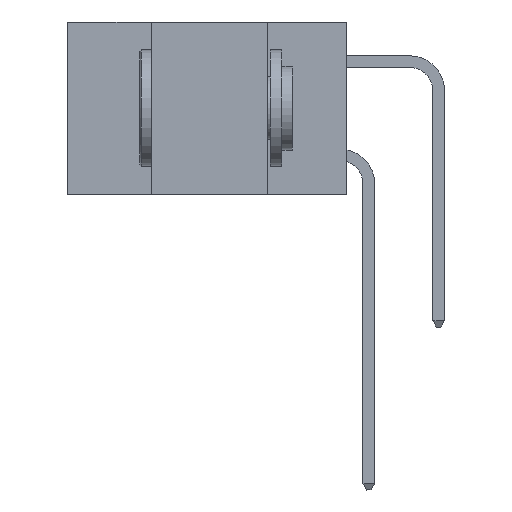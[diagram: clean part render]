
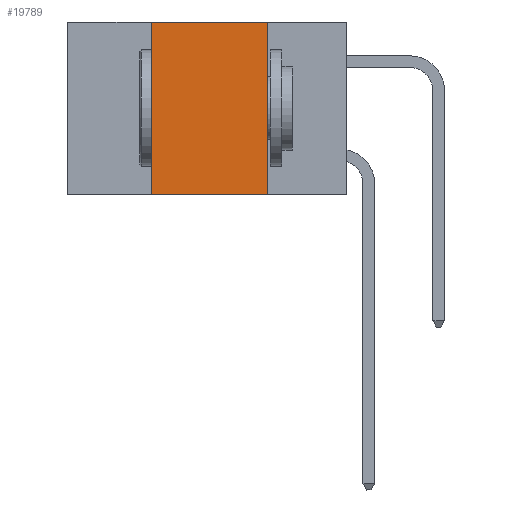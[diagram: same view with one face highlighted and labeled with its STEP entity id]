
A CAD part, left-side view. The second image highlights one B-rep face of the part: STEP entity #19789.
In plain terms, the highlighted planar face has unit normal (-1, 0, 0).
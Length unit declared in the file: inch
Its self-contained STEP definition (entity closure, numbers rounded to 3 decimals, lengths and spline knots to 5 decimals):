
#940 = VERTEX_POINT ( 'NONE', #16587 ) ;
#1524 = EDGE_LOOP ( 'NONE', ( #10080, #21370, #4394, #13162 ) ) ;
#1632 = VERTEX_POINT ( 'NONE', #16380 ) ;
#4146 = LINE ( 'NONE', #13945, #11488 ) ;
#4394 = ORIENTED_EDGE ( 'NONE', *, *, #10750, .F. ) ;
#5174 = DIRECTION ( 'NONE',  ( 0., 0., 1. ) ) ;
#5801 = DIRECTION ( 'NONE',  ( 0., 0., -1. ) ) ;
#6802 = LINE ( 'NONE', #19123, #24147 ) ;
#8670 = CARTESIAN_POINT ( 'NONE',  ( 0., 0.6, -0.37 ) ) ;
#10080 = ORIENTED_EDGE ( 'NONE', *, *, #20058, .F. ) ;
#10750 = EDGE_CURVE ( 'NONE', #1632, #17038, #4146, .T. ) ;
#10974 = VECTOR ( 'NONE', #13246, 39.37008 ) ;
#10980 = CARTESIAN_POINT ( 'NONE',  ( 0., 0.6, 0. ) ) ;
#11488 = VECTOR ( 'NONE', #5174, 39.37008 ) ;
#11747 = EDGE_CURVE ( 'NONE', #17038, #15437, #12355, .T. ) ;
#12355 = LINE ( 'NONE', #10980, #10974 ) ;
#13162 = ORIENTED_EDGE ( 'NONE', *, *, #15698, .T. ) ;
#13246 = DIRECTION ( 'NONE',  ( 0., -1., 0. ) ) ;
#13945 = CARTESIAN_POINT ( 'NONE',  ( 0., 0.42, 0. ) ) ;
#15437 = VERTEX_POINT ( 'NONE', #22383 ) ;
#15698 = EDGE_CURVE ( 'NONE', #1632, #940, #17795, .T. ) ;
#16380 = CARTESIAN_POINT ( 'NONE',  ( 0., 0.42, -0.37 ) ) ;
#16527 = AXIS2_PLACEMENT_3D ( 'NONE', #26536, #26274, #5801 ) ;
#16587 = CARTESIAN_POINT ( 'NONE',  ( 0., 0.17, -0.37 ) ) ;
#17038 = VERTEX_POINT ( 'NONE', #17997 ) ;
#17795 = LINE ( 'NONE', #8670, #19151 ) ;
#17997 = CARTESIAN_POINT ( 'NONE',  ( 0., 0.42, 0. ) ) ;
#19123 = CARTESIAN_POINT ( 'NONE',  ( 0., 0.17, 0. ) ) ;
#19151 = VECTOR ( 'NONE', #23626, 39.37008 ) ;
#19789 = ADVANCED_FACE ( 'NONE', ( #25503 ), #20559, .F. ) ;
#20058 = EDGE_CURVE ( 'NONE', #15437, #940, #6802, .T. ) ;
#20559 = PLANE ( 'NONE',  #16527 ) ;
#21370 = ORIENTED_EDGE ( 'NONE', *, *, #11747, .F. ) ;
#22383 = CARTESIAN_POINT ( 'NONE',  ( 0., 0.17, 0. ) ) ;
#23489 = DIRECTION ( 'NONE',  ( 0., 0., -1. ) ) ;
#23626 = DIRECTION ( 'NONE',  ( 0., -1., 0. ) ) ;
#24147 = VECTOR ( 'NONE', #23489, 39.37008 ) ;
#25503 = FACE_OUTER_BOUND ( 'NONE', #1524, .T. ) ;
#26274 = DIRECTION ( 'NONE',  ( 1., 0., 0. ) ) ;
#26536 = CARTESIAN_POINT ( 'NONE',  ( 0., 0.6, 0. ) ) ;
